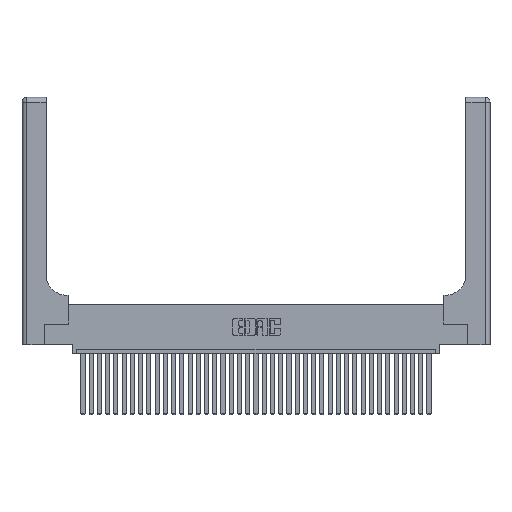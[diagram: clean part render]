
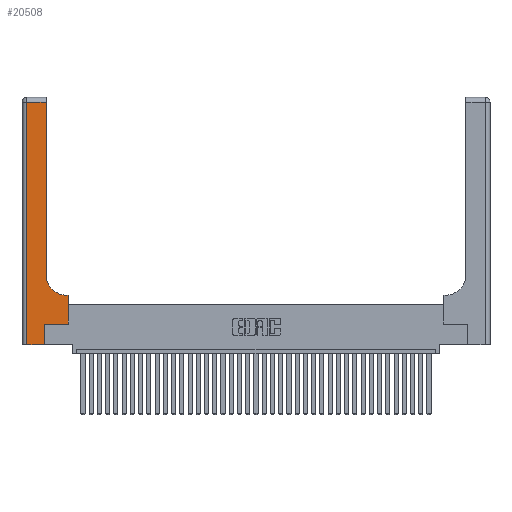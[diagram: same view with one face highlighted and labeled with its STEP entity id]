
A CAD part, top view. The second image highlights one B-rep face of the part: STEP entity #20508.
In plain terms, the highlighted planar face has unit normal (0, 0, 1).
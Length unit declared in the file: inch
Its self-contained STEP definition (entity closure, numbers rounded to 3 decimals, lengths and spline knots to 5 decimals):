
#496 = CARTESIAN_POINT ( 'NONE',  ( 0.5585, 0.25, 0.37 ) ) ;
#909 = CARTESIAN_POINT ( 'NONE',  ( 0.2915, 0.85, 0.37 ) ) ;
#1249 = EDGE_CURVE ( 'NONE', #31061, #6126, #19859, .T. ) ;
#2920 = VECTOR ( 'NONE', #23518, 39.37008 ) ;
#3037 = VERTEX_POINT ( 'NONE', #3866 ) ;
#3203 = DIRECTION ( 'NONE',  ( 0., 1., 0. ) ) ;
#3840 = CARTESIAN_POINT ( 'NONE',  ( 0., 0., 0.37 ) ) ;
#3866 = CARTESIAN_POINT ( 'NONE',  ( 0.5585, 0.25, 0.37 ) ) ;
#4282 = DIRECTION ( 'NONE',  ( -1., 0., 0. ) ) ;
#4999 = EDGE_CURVE ( 'NONE', #3037, #23044, #29442, .T. ) ;
#5487 = LINE ( 'NONE', #5844, #36206 ) ;
#5844 = CARTESIAN_POINT ( 'NONE',  ( 0.269, 0., 0.37 ) ) ;
#5869 = DIRECTION ( 'NONE',  ( 1., 0., 0. ) ) ;
#6126 = VERTEX_POINT ( 'NONE', #35182 ) ;
#6526 = CARTESIAN_POINT ( 'NONE',  ( 0.5415, 0.6, 0.37 ) ) ;
#6790 = CARTESIAN_POINT ( 'NONE',  ( 0., 2.94, 0.37 ) ) ;
#7161 = ORIENTED_EDGE ( 'NONE', *, *, #19403, .T. ) ;
#7690 = LINE ( 'NONE', #12215, #10394 ) ;
#8936 = CARTESIAN_POINT ( 'NONE',  ( 0.06, 3., 0.37 ) ) ;
#9719 = PLANE ( 'NONE',  #31795 ) ;
#10092 = EDGE_CURVE ( 'NONE', #6126, #28454, #26491, .T. ) ;
#10320 = VECTOR ( 'NONE', #14708, 39.37008 ) ;
#10394 = VECTOR ( 'NONE', #15154, 39.37008 ) ;
#10870 = VERTEX_POINT ( 'NONE', #15955 ) ;
#12132 = AXIS2_PLACEMENT_3D ( 'NONE', #31759, #14855, #14503 ) ;
#12215 = CARTESIAN_POINT ( 'NONE',  ( 0.2915, 0.6, 0.37 ) ) ;
#12568 = DIRECTION ( 'NONE',  ( 0., 0., -1. ) ) ;
#13072 = CARTESIAN_POINT ( 'NONE',  ( 0.269, 0., 0.37 ) ) ;
#13252 = DIRECTION ( 'NONE',  ( 0., 1., 0. ) ) ;
#13255 = ORIENTED_EDGE ( 'NONE', *, *, #23567, .T. ) ;
#13400 = VECTOR ( 'NONE', #13252, 39.37008 ) ;
#14503 = DIRECTION ( 'NONE',  ( 1., 0., 0. ) ) ;
#14591 = ORIENTED_EDGE ( 'NONE', *, *, #4999, .T. ) ;
#14686 = ORIENTED_EDGE ( 'NONE', *, *, #22269, .T. ) ;
#14708 = DIRECTION ( 'NONE',  ( 0., -1., 0. ) ) ;
#14855 = DIRECTION ( 'NONE',  ( 0., 0., -1. ) ) ;
#14991 = CARTESIAN_POINT ( 'NONE',  ( 0., 3., 0.37 ) ) ;
#15154 = DIRECTION ( 'NONE',  ( -1., 0., 0. ) ) ;
#15955 = CARTESIAN_POINT ( 'NONE',  ( 0.269, 0.25, 0.37 ) ) ;
#17215 = CARTESIAN_POINT ( 'NONE',  ( 0.06, 0., 0.37 ) ) ;
#17560 = VECTOR ( 'NONE', #5869, 39.37008 ) ;
#17815 = FACE_OUTER_BOUND ( 'NONE', #28260, .T. ) ;
#18392 = LINE ( 'NONE', #24233, #13400 ) ;
#19403 = EDGE_CURVE ( 'NONE', #27532, #31061, #18392, .T. ) ;
#19859 = LINE ( 'NONE', #6790, #34714 ) ;
#19869 = VERTEX_POINT ( 'NONE', #13072 ) ;
#20508 = ADVANCED_FACE ( 'NONE', ( #17815 ), #9719, .F. ) ;
#21253 = DIRECTION ( 'NONE',  ( 1., 0., 0. ) ) ;
#21647 = LINE ( 'NONE', #31698, #17560 ) ;
#21901 = EDGE_CURVE ( 'NONE', #28454, #19869, #32086, .T. ) ;
#22269 = EDGE_CURVE ( 'NONE', #19869, #10870, #5487, .T. ) ;
#23044 = VERTEX_POINT ( 'NONE', #29076 ) ;
#23227 = VERTEX_POINT ( 'NONE', #6526 ) ;
#23518 = DIRECTION ( 'NONE',  ( 0., 1., 0. ) ) ;
#23567 = EDGE_CURVE ( 'NONE', #10870, #3037, #21647, .T. ) ;
#24233 = CARTESIAN_POINT ( 'NONE',  ( 0.2915, 3., 0.37 ) ) ;
#24835 = CARTESIAN_POINT ( 'NONE',  ( 0.2915, 2.94, 0.37 ) ) ;
#26491 = LINE ( 'NONE', #8936, #10320 ) ;
#26586 = ORIENTED_EDGE ( 'NONE', *, *, #1249, .T. ) ;
#27532 = VERTEX_POINT ( 'NONE', #909 ) ;
#28260 = EDGE_LOOP ( 'NONE', ( #7161, #26586, #34771, #36984, #14686, #13255, #14591, #34889, #32689 ) ) ;
#28454 = VERTEX_POINT ( 'NONE', #17215 ) ;
#29076 = CARTESIAN_POINT ( 'NONE',  ( 0.5585, 0.6, 0.37 ) ) ;
#29442 = LINE ( 'NONE', #496, #2920 ) ;
#29980 = DIRECTION ( 'NONE',  ( -1., 0., 0. ) ) ;
#30709 = CIRCLE ( 'NONE', #12132, 0.25 ) ;
#31061 = VERTEX_POINT ( 'NONE', #24835 ) ;
#31698 = CARTESIAN_POINT ( 'NONE',  ( 0.269, 0.25, 0.37 ) ) ;
#31759 = CARTESIAN_POINT ( 'NONE',  ( 0.5415, 0.85, 0.37 ) ) ;
#31795 = AXIS2_PLACEMENT_3D ( 'NONE', #14991, #12568, #29980 ) ;
#32086 = LINE ( 'NONE', #3840, #36688 ) ;
#32689 = ORIENTED_EDGE ( 'NONE', *, *, #33426, .T. ) ;
#32969 = EDGE_CURVE ( 'NONE', #23044, #23227, #7690, .T. ) ;
#33426 = EDGE_CURVE ( 'NONE', #23227, #27532, #30709, .T. ) ;
#34714 = VECTOR ( 'NONE', #4282, 39.37008 ) ;
#34771 = ORIENTED_EDGE ( 'NONE', *, *, #10092, .T. ) ;
#34889 = ORIENTED_EDGE ( 'NONE', *, *, #32969, .T. ) ;
#35182 = CARTESIAN_POINT ( 'NONE',  ( 0.06, 2.94, 0.37 ) ) ;
#36206 = VECTOR ( 'NONE', #3203, 39.37008 ) ;
#36688 = VECTOR ( 'NONE', #21253, 39.37008 ) ;
#36984 = ORIENTED_EDGE ( 'NONE', *, *, #21901, .T. ) ;
